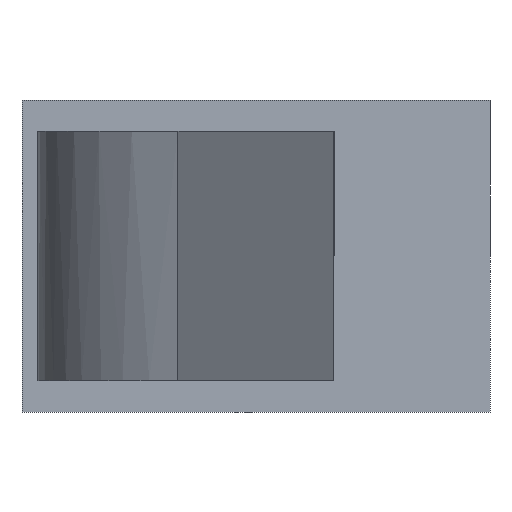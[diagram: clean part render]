
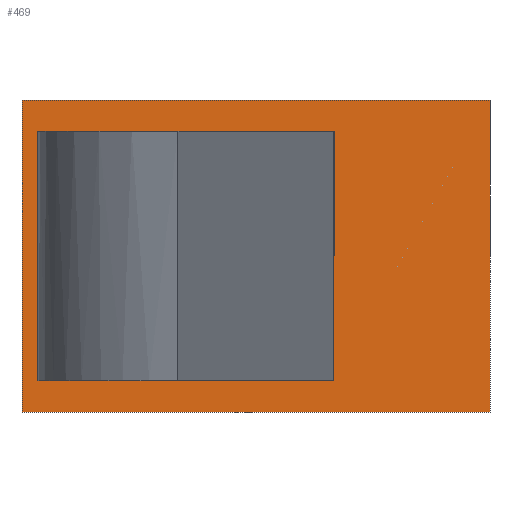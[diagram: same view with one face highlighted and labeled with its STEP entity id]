
A CAD part, left-side view. The second image highlights one B-rep face of the part: STEP entity #469.
In plain terms, the highlighted planar face has unit normal (-1, 0, 0).
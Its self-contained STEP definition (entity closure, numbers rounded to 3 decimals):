
#23 = DIRECTION ( 'NONE',  ( 0., -1., 0. ) ) ;
#34 = VERTEX_POINT ( 'NONE', #144 ) ;
#42 = AXIS2_PLACEMENT_3D ( 'NONE', #302, #66, #349 ) ;
#44 = VERTEX_POINT ( 'NONE', #373 ) ;
#66 = DIRECTION ( 'NONE',  ( 1., 0., 0. ) ) ;
#68 = VERTEX_POINT ( 'NONE', #234 ) ;
#71 = EDGE_CURVE ( 'NONE', #534, #305, #486, .T. ) ;
#89 = EDGE_CURVE ( 'NONE', #305, #44, #475, .T. ) ;
#92 = CARTESIAN_POINT ( 'NONE',  ( 4., 1.25, 2. ) ) ;
#97 = EDGE_CURVE ( 'NONE', #347, #344, #485, .T. ) ;
#98 = ORIENTED_EDGE ( 'NONE', *, *, #342, .T. ) ;
#109 = DIRECTION ( 'NONE',  ( 0., -1., 0. ) ) ;
#117 = EDGE_CURVE ( 'NONE', #34, #347, #455, .T. ) ;
#118 = CARTESIAN_POINT ( 'NONE',  ( 4., 0., -2.5 ) ) ;
#121 = CARTESIAN_POINT ( 'NONE',  ( 4., 6.25, -2.5 ) ) ;
#123 = DIRECTION ( 'NONE',  ( 0., 0., 1. ) ) ;
#124 = VERTEX_POINT ( 'NONE', #149 ) ;
#131 = ORIENTED_EDGE ( 'NONE', *, *, #263, .F. ) ;
#136 = DIRECTION ( 'NONE',  ( 0., 1., 0. ) ) ;
#144 = CARTESIAN_POINT ( 'NONE',  ( 4., 4.574, -2. ) ) ;
#149 = CARTESIAN_POINT ( 'NONE',  ( 4., 6.25, 2.5 ) ) ;
#154 = DIRECTION ( 'NONE',  ( 0., -1., 0. ) ) ;
#159 = CARTESIAN_POINT ( 'NONE',  ( 4., 4.574, 2. ) ) ;
#167 = ORIENTED_EDGE ( 'NONE', *, *, #283, .F. ) ;
#175 = CARTESIAN_POINT ( 'NONE',  ( 4., -1.25, -2.5 ) ) ;
#176 = DIRECTION ( 'NONE',  ( 0., 0., 1. ) ) ;
#197 = CARTESIAN_POINT ( 'NONE',  ( 4., 4.574, -2.501 ) ) ;
#234 = CARTESIAN_POINT ( 'NONE',  ( 4., 1.25, -2. ) ) ;
#263 = EDGE_CURVE ( 'NONE', #34, #68, #413, .T. ) ;
#280 = DIRECTION ( 'NONE',  ( 0., 0., 1. ) ) ;
#283 = EDGE_CURVE ( 'NONE', #534, #124, #408, .T. ) ;
#295 = CARTESIAN_POINT ( 'NONE',  ( 4., 6.25, 2. ) ) ;
#296 = CARTESIAN_POINT ( 'NONE',  ( 4., 1.25, -2.501 ) ) ;
#302 = CARTESIAN_POINT ( 'NONE',  ( 4., 0., -2.501 ) ) ;
#305 = VERTEX_POINT ( 'NONE', #175 ) ;
#309 = CARTESIAN_POINT ( 'NONE',  ( 4., 6.25, -2. ) ) ;
#341 = CARTESIAN_POINT ( 'NONE',  ( 4., 6.25, -2.501 ) ) ;
#342 = EDGE_CURVE ( 'NONE', #344, #68, #404, .T. ) ;
#344 = VERTEX_POINT ( 'NONE', #92 ) ;
#347 = VERTEX_POINT ( 'NONE', #159 ) ;
#348 = LINE ( 'NONE', #393, #350 ) ;
#349 = DIRECTION ( 'NONE',  ( 0., 0., -1. ) ) ;
#350 = VECTOR ( 'NONE', #136, 1000. ) ;
#357 = FACE_BOUND ( 'NONE', #531, .T. ) ;
#359 = FACE_OUTER_BOUND ( 'NONE', #398, .T. ) ;
#373 = CARTESIAN_POINT ( 'NONE',  ( 4., -1.25, 2.5 ) ) ;
#379 = CARTESIAN_POINT ( 'NONE',  ( 4., -1.25, -2.5 ) ) ;
#380 = VECTOR ( 'NONE', #154, 1000. ) ;
#389 = ORIENTED_EDGE ( 'NONE', *, *, #97, .T. ) ;
#393 = CARTESIAN_POINT ( 'NONE',  ( 4., 0., 2.5 ) ) ;
#397 = VECTOR ( 'NONE', #176, 1000. ) ;
#398 = EDGE_LOOP ( 'NONE', ( #492, #525, #419, #167 ) ) ;
#401 = VECTOR ( 'NONE', #499, 1000. ) ;
#404 = LINE ( 'NONE', #296, #401 ) ;
#408 = LINE ( 'NONE', #341, #397 ) ;
#413 = LINE ( 'NONE', #309, #435 ) ;
#419 = ORIENTED_EDGE ( 'NONE', *, *, #477, .T. ) ;
#435 = VECTOR ( 'NONE', #109, 1000. ) ;
#451 = VECTOR ( 'NONE', #280, 1000. ) ;
#455 = LINE ( 'NONE', #197, #451 ) ;
#469 = ADVANCED_FACE ( 'NONE', ( #359, #357 ), #479, .F. ) ;
#473 = VECTOR ( 'NONE', #123, 1000. ) ;
#475 = LINE ( 'NONE', #379, #473 ) ;
#477 = EDGE_CURVE ( 'NONE', #44, #124, #348, .T. ) ;
#479 = PLANE ( 'NONE',  #42 ) ;
#485 = LINE ( 'NONE', #295, #380 ) ;
#486 = LINE ( 'NONE', #118, #491 ) ;
#491 = VECTOR ( 'NONE', #23, 1000. ) ;
#492 = ORIENTED_EDGE ( 'NONE', *, *, #71, .T. ) ;
#499 = DIRECTION ( 'NONE',  ( 0., 0., -1. ) ) ;
#510 = ORIENTED_EDGE ( 'NONE', *, *, #117, .T. ) ;
#525 = ORIENTED_EDGE ( 'NONE', *, *, #89, .T. ) ;
#531 = EDGE_LOOP ( 'NONE', ( #98, #131, #510, #389 ) ) ;
#534 = VERTEX_POINT ( 'NONE', #121 ) ;
